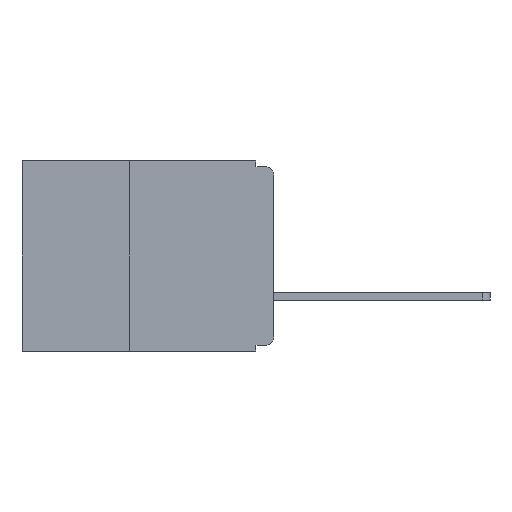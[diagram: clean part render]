
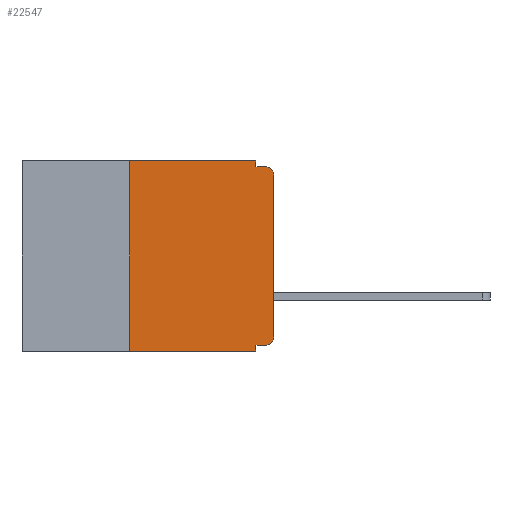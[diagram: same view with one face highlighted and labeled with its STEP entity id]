
A CAD part, left-side view. The second image highlights one B-rep face of the part: STEP entity #22547.
In plain terms, the highlighted planar face has unit normal (-1, 0, 0).
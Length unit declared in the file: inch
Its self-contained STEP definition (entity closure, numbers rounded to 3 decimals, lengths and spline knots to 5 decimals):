
#34 = VECTOR ( 'NONE', #107, 39.37008 ) ;
#107 = DIRECTION ( 'NONE',  ( 0., 0., -1. ) ) ;
#178 = EDGE_CURVE ( 'NONE', #26005, #11954, #20406, .T. ) ;
#179 = DIRECTION ( 'NONE',  ( 0., 0., -1. ) ) ;
#782 = LINE ( 'NONE', #21605, #34 ) ;
#2104 = EDGE_CURVE ( 'NONE', #12541, #16474, #22108, .T. ) ;
#2137 = DIRECTION ( 'NONE',  ( 0., -1., 0. ) ) ;
#2142 = VECTOR ( 'NONE', #11942, 39.37008 ) ;
#2428 = VECTOR ( 'NONE', #5546, 39.37008 ) ;
#2758 = DIRECTION ( 'NONE',  ( 0., 1., 0. ) ) ;
#2929 = AXIS2_PLACEMENT_3D ( 'NONE', #12172, #14526, #179 ) ;
#3145 = ORIENTED_EDGE ( 'NONE', *, *, #26753, .T. ) ;
#3219 = CARTESIAN_POINT ( 'NONE',  ( 0., 0.031, -0.32 ) ) ;
#3879 = CARTESIAN_POINT ( 'NONE',  ( 0., 0., 0. ) ) ;
#4499 = DIRECTION ( 'NONE',  ( 0., 0., 1. ) ) ;
#5057 = ORIENTED_EDGE ( 'NONE', *, *, #15460, .T. ) ;
#5305 = ORIENTED_EDGE ( 'NONE', *, *, #16556, .F. ) ;
#5546 = DIRECTION ( 'NONE',  ( 0., -1., 0. ) ) ;
#5593 = ORIENTED_EDGE ( 'NONE', *, *, #178, .F. ) ;
#5598 = LINE ( 'NONE', #19848, #30020 ) ;
#5746 = VECTOR ( 'NONE', #29977, 39.37008 ) ;
#6235 = LINE ( 'NONE', #6930, #24381 ) ;
#6930 = CARTESIAN_POINT ( 'NONE',  ( 0., 0.437, 0. ) ) ;
#7215 = LINE ( 'NONE', #3879, #5746 ) ;
#7902 = EDGE_CURVE ( 'NONE', #12541, #18085, #9161, .T. ) ;
#8455 = CIRCLE ( 'NONE', #26206, 0.015 ) ;
#8855 = CARTESIAN_POINT ( 'NONE',  ( 0., 0., -0.025 ) ) ;
#9161 = LINE ( 'NONE', #18751, #27274 ) ;
#9254 = CIRCLE ( 'NONE', #22513, 0.015 ) ;
#9273 = CARTESIAN_POINT ( 'NONE',  ( 0., 0., -0.305 ) ) ;
#9328 = DIRECTION ( 'NONE',  ( 0., -1., 0. ) ) ;
#9774 = PLANE ( 'NONE',  #2929 ) ;
#9778 = EDGE_CURVE ( 'NONE', #22066, #16474, #782, .T. ) ;
#11530 = CARTESIAN_POINT ( 'NONE',  ( 0., 0.015, -0.025 ) ) ;
#11594 = ORIENTED_EDGE ( 'NONE', *, *, #2104, .T. ) ;
#11942 = DIRECTION ( 'NONE',  ( 0., 0., -1. ) ) ;
#11954 = VERTEX_POINT ( 'NONE', #30349 ) ;
#12172 = CARTESIAN_POINT ( 'NONE',  ( 0., 0.437, 0. ) ) ;
#12231 = CARTESIAN_POINT ( 'NONE',  ( 0., 0.25, 0. ) ) ;
#12541 = VERTEX_POINT ( 'NONE', #13724 ) ;
#13287 = CARTESIAN_POINT ( 'NONE',  ( 0., 0.015, -0.305 ) ) ;
#13724 = CARTESIAN_POINT ( 'NONE',  ( 0., 0.25, -0.33 ) ) ;
#13881 = DIRECTION ( 'NONE',  ( 0., 0., -1. ) ) ;
#14424 = ORIENTED_EDGE ( 'NONE', *, *, #9778, .F. ) ;
#14526 = DIRECTION ( 'NONE',  ( 1., 0., 0. ) ) ;
#15010 = VERTEX_POINT ( 'NONE', #8855 ) ;
#15397 = ORIENTED_EDGE ( 'NONE', *, *, #23034, .F. ) ;
#15460 = EDGE_CURVE ( 'NONE', #28847, #23509, #9254, .T. ) ;
#15689 = DIRECTION ( 'NONE',  ( 0., 0., -1. ) ) ;
#16474 = VERTEX_POINT ( 'NONE', #21916 ) ;
#16484 = CARTESIAN_POINT ( 'NONE',  ( 0., 0.015, -0.01 ) ) ;
#16556 = EDGE_CURVE ( 'NONE', #11954, #28188, #22139, .T. ) ;
#17372 = CARTESIAN_POINT ( 'NONE',  ( 0., 0., -0.01 ) ) ;
#18043 = ORIENTED_EDGE ( 'NONE', *, *, #22958, .T. ) ;
#18085 = VERTEX_POINT ( 'NONE', #12231 ) ;
#18090 = ORIENTED_EDGE ( 'NONE', *, *, #7902, .F. ) ;
#18751 = CARTESIAN_POINT ( 'NONE',  ( 0., 0.25, -0.33 ) ) ;
#19848 = CARTESIAN_POINT ( 'NONE',  ( 0., 0., -0.32 ) ) ;
#19946 = CARTESIAN_POINT ( 'NONE',  ( 0., 0.031, 0. ) ) ;
#20406 = LINE ( 'NONE', #19946, #2142 ) ;
#20683 = EDGE_CURVE ( 'NONE', #28847, #22066, #5598, .T. ) ;
#21392 = ORIENTED_EDGE ( 'NONE', *, *, #20683, .F. ) ;
#21605 = CARTESIAN_POINT ( 'NONE',  ( 0., 0.031, -0.33 ) ) ;
#21916 = CARTESIAN_POINT ( 'NONE',  ( 0., 0.031, -0.33 ) ) ;
#22066 = VERTEX_POINT ( 'NONE', #3219 ) ;
#22108 = LINE ( 'NONE', #26663, #27632 ) ;
#22139 = LINE ( 'NONE', #17372, #2428 ) ;
#22513 = AXIS2_PLACEMENT_3D ( 'NONE', #13287, #29813, #15689 ) ;
#22547 = ADVANCED_FACE ( 'NONE', ( #25885 ), #9774, .F. ) ;
#22958 = EDGE_CURVE ( 'NONE', #15010, #28188, #8455, .T. ) ;
#23034 = EDGE_CURVE ( 'NONE', #18085, #26005, #6235, .T. ) ;
#23509 = VERTEX_POINT ( 'NONE', #9273 ) ;
#24381 = VECTOR ( 'NONE', #9328, 39.37008 ) ;
#25844 = EDGE_LOOP ( 'NONE', ( #3145, #18043, #5305, #5593, #15397, #18090, #11594, #14424, #21392, #5057 ) ) ;
#25885 = FACE_OUTER_BOUND ( 'NONE', #25844, .T. ) ;
#26005 = VERTEX_POINT ( 'NONE', #26384 ) ;
#26206 = AXIS2_PLACEMENT_3D ( 'NONE', #11530, #28039, #13881 ) ;
#26357 = CARTESIAN_POINT ( 'NONE',  ( 0., 0.015, -0.32 ) ) ;
#26384 = CARTESIAN_POINT ( 'NONE',  ( 0., 0.031, 0. ) ) ;
#26663 = CARTESIAN_POINT ( 'NONE',  ( 0., 0.437, -0.33 ) ) ;
#26753 = EDGE_CURVE ( 'NONE', #23509, #15010, #7215, .T. ) ;
#27274 = VECTOR ( 'NONE', #4499, 39.37008 ) ;
#27632 = VECTOR ( 'NONE', #2137, 39.37008 ) ;
#28039 = DIRECTION ( 'NONE',  ( -1., 0., 0. ) ) ;
#28188 = VERTEX_POINT ( 'NONE', #16484 ) ;
#28847 = VERTEX_POINT ( 'NONE', #26357 ) ;
#29813 = DIRECTION ( 'NONE',  ( -1., 0., 0. ) ) ;
#29977 = DIRECTION ( 'NONE',  ( 0., 0., 1. ) ) ;
#30020 = VECTOR ( 'NONE', #2758, 39.37008 ) ;
#30349 = CARTESIAN_POINT ( 'NONE',  ( 0., 0.031, -0.01 ) ) ;
